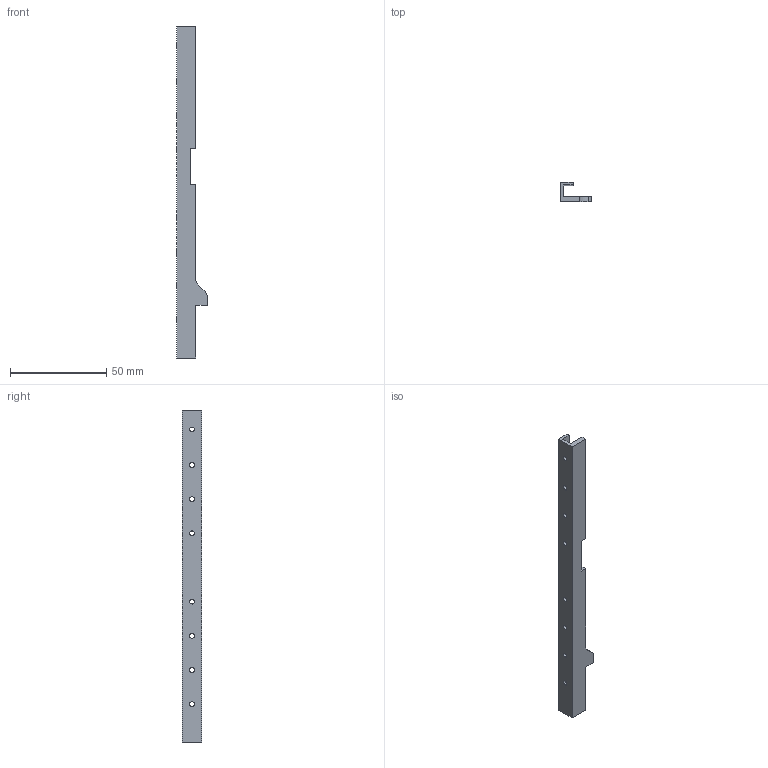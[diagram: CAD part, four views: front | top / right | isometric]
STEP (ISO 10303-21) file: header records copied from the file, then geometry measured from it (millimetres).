
FILE_DESCRIPTION(/* description */ (''),/* implementation_level */ '2;1');
FILE_NAME(/* name */ 'Plastikov Left Rail Milled Spec v3.0.stp',/* time_stamp */ '2021-10-04T20:44:11-05:00',/* author */ ('johne'),/* organization */ (''),/* preprocessor_version */ 'ST-DEVELOPER v18.1',/* originating_system */ 'Autodesk Inventor 2020',/* authorisation */ '');
FILE_SCHEMA (('AUTOMOTIVE_DESIGN { 1 0 10303 214 3 1 1 }'));
Length unit declared in the file: inch
Products named in the file (1): Plastikov Left Rail Milled Spec v2.1
Bounding box: 15.75 x 10 x 172.77 mm (x, y, z)
Volume: 7608.9 mm3; surface area: 8681.8 mm2
Topology: 1 solids, 1 shells, 27 faces, 83 edges, 58 vertices
Faces by surface type: plane 17, cylinder 10
Full cylindrical faces by diameter (mm): 2.5 x8
Entity records: 1024 total; most frequent: CARTESIAN_POINT 169, DIRECTION 167, ORIENTED_EDGE 166, EDGE_CURVE 83, VERTEX_POINT 58, AXIS2_PLACEMENT_3D 56, LINE 55, VECTOR 55
